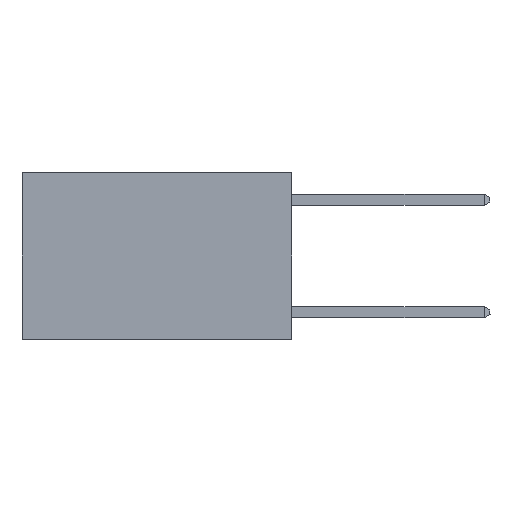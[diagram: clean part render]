
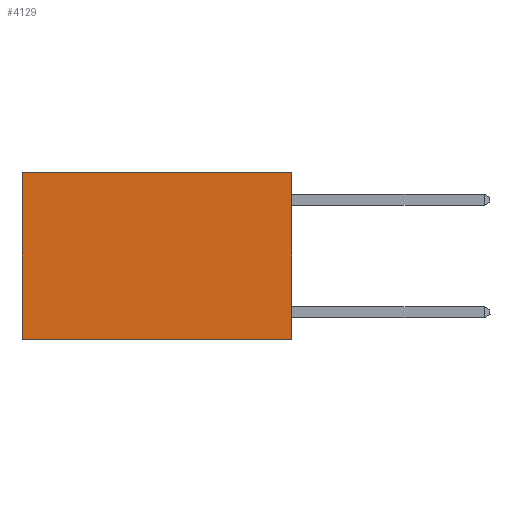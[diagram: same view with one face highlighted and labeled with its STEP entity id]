
A CAD part, left-side view. The second image highlights one B-rep face of the part: STEP entity #4129.
In plain terms, the highlighted planar face has unit normal (-1, 0, 0).
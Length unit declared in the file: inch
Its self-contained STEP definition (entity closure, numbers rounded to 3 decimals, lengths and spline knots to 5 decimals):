
#188 = AXIS2_PLACEMENT_3D ( 'NONE', #9011, #10694, #5659 ) ;
#637 = LINE ( 'NONE', #3329, #5152 ) ;
#970 = DIRECTION ( 'NONE',  ( 0., 1., 0. ) ) ;
#1688 = CARTESIAN_POINT ( 'NONE',  ( 0.2625, 0.6, 0. ) ) ;
#2134 = VERTEX_POINT ( 'NONE', #4671 ) ;
#2380 = LINE ( 'NONE', #6314, #9306 ) ;
#2431 = CARTESIAN_POINT ( 'NONE',  ( 0.2625, 0., -0.37 ) ) ;
#2528 = VECTOR ( 'NONE', #8520, 39.37008 ) ;
#2815 = VERTEX_POINT ( 'NONE', #8156 ) ;
#3329 = CARTESIAN_POINT ( 'NONE',  ( 0.2625, 0., 0. ) ) ;
#3439 = VERTEX_POINT ( 'NONE', #5541 ) ;
#3646 = VECTOR ( 'NONE', #11122, 39.37008 ) ;
#4129 = ADVANCED_FACE ( 'NONE', ( #5419 ), #9049, .F. ) ;
#4671 = CARTESIAN_POINT ( 'NONE',  ( 0.2625, 0.6, -0.37 ) ) ;
#5152 = VECTOR ( 'NONE', #11010, 39.37008 ) ;
#5419 = FACE_OUTER_BOUND ( 'NONE', #6409, .T. ) ;
#5541 = CARTESIAN_POINT ( 'NONE',  ( 0.2625, 0., 0. ) ) ;
#5659 = DIRECTION ( 'NONE',  ( 0., 0., -1. ) ) ;
#5912 = EDGE_CURVE ( 'NONE', #9691, #2134, #10469, .T. ) ;
#6314 = CARTESIAN_POINT ( 'NONE',  ( 0.2625, 0., 0. ) ) ;
#6409 = EDGE_LOOP ( 'NONE', ( #6693, #6717, #6754, #6789 ) ) ;
#6463 = EDGE_CURVE ( 'NONE', #2815, #2134, #9447, .T. ) ;
#6693 = ORIENTED_EDGE ( 'NONE', *, *, #5912, .T. ) ;
#6717 = ORIENTED_EDGE ( 'NONE', *, *, #6463, .F. ) ;
#6739 = EDGE_CURVE ( 'NONE', #3439, #9691, #2380, .T. ) ;
#6754 = ORIENTED_EDGE ( 'NONE', *, *, #8222, .F. ) ;
#6789 = ORIENTED_EDGE ( 'NONE', *, *, #6739, .T. ) ;
#7350 = CARTESIAN_POINT ( 'NONE',  ( 0.2625, 0.6, 0. ) ) ;
#8156 = CARTESIAN_POINT ( 'NONE',  ( 0.2625, 0., -0.37 ) ) ;
#8222 = EDGE_CURVE ( 'NONE', #3439, #2815, #637, .T. ) ;
#8520 = DIRECTION ( 'NONE',  ( 0., 1., 0. ) ) ;
#9011 = CARTESIAN_POINT ( 'NONE',  ( 0.2625, 0., 0. ) ) ;
#9049 = PLANE ( 'NONE',  #188 ) ;
#9306 = VECTOR ( 'NONE', #970, 39.37008 ) ;
#9447 = LINE ( 'NONE', #2431, #2528 ) ;
#9691 = VERTEX_POINT ( 'NONE', #7350 ) ;
#10469 = LINE ( 'NONE', #1688, #3646 ) ;
#10694 = DIRECTION ( 'NONE',  ( 1., 0., 0. ) ) ;
#11010 = DIRECTION ( 'NONE',  ( 0., 0., -1. ) ) ;
#11122 = DIRECTION ( 'NONE',  ( 0., 0., -1. ) ) ;
